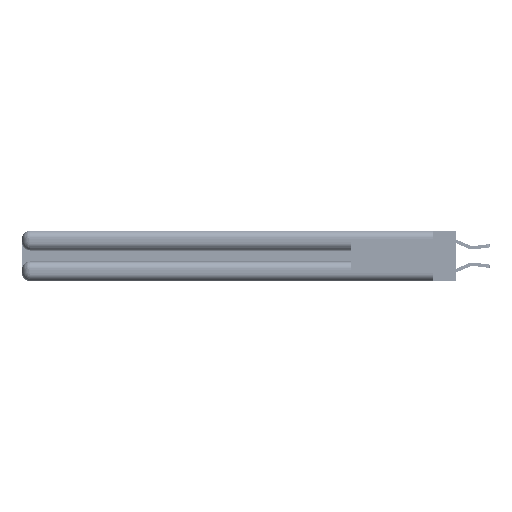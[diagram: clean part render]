
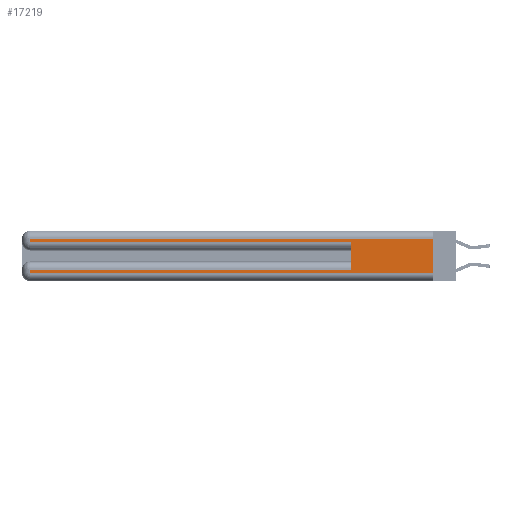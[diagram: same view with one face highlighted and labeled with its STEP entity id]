
A CAD part, left-side view. The second image highlights one B-rep face of the part: STEP entity #17219.
In plain terms, the highlighted planar face has unit normal (-1, 0, 0).
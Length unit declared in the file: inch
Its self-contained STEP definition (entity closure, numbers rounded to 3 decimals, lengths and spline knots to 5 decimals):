
#567 = CARTESIAN_POINT ( 'NONE',  ( 0., 2.94, 0.06 ) ) ;
#1386 = ORIENTED_EDGE ( 'NONE', *, *, #13064, .T. ) ;
#1607 = CARTESIAN_POINT ( 'NONE',  ( 0., 0.6, 0.145 ) ) ;
#2056 = VECTOR ( 'NONE', #31576, 39.37008 ) ;
#3484 = DIRECTION ( 'NONE',  ( 0., 1., 0. ) ) ;
#3649 = DIRECTION ( 'NONE',  ( 1., 0., 0. ) ) ;
#3768 = VERTEX_POINT ( 'NONE', #10625 ) ;
#4222 = LINE ( 'NONE', #1607, #11592 ) ;
#4477 = ORIENTED_EDGE ( 'NONE', *, *, #33767, .T. ) ;
#4599 = DIRECTION ( 'NONE',  ( 0., 0., -1. ) ) ;
#4734 = ORIENTED_EDGE ( 'NONE', *, *, #36542, .T. ) ;
#5939 = LINE ( 'NONE', #31522, #25085 ) ;
#6443 = LINE ( 'NONE', #23136, #7907 ) ;
#6954 = VERTEX_POINT ( 'NONE', #567 ) ;
#7397 = CARTESIAN_POINT ( 'NONE',  ( 0., 0.6, 0.285 ) ) ;
#7907 = VECTOR ( 'NONE', #3484, 39.37008 ) ;
#9080 = DIRECTION ( 'NONE',  ( 0., -1., 0. ) ) ;
#9557 = FACE_OUTER_BOUND ( 'NONE', #30323, .T. ) ;
#10322 = CARTESIAN_POINT ( 'NONE',  ( 0., 0., 0.31 ) ) ;
#10553 = VERTEX_POINT ( 'NONE', #7397 ) ;
#10625 = CARTESIAN_POINT ( 'NONE',  ( 0., 0.6, 0.085 ) ) ;
#11592 = VECTOR ( 'NONE', #26823, 39.37008 ) ;
#11743 = LINE ( 'NONE', #28624, #2056 ) ;
#11820 = PLANE ( 'NONE',  #14605 ) ;
#12938 = LINE ( 'NONE', #10322, #17382 ) ;
#12982 = EDGE_CURVE ( 'NONE', #3768, #16182, #6443, .T. ) ;
#13064 = EDGE_CURVE ( 'NONE', #24752, #29821, #12938, .T. ) ;
#13301 = LINE ( 'NONE', #30186, #20770 ) ;
#14605 = AXIS2_PLACEMENT_3D ( 'NONE', #34790, #3649, #20668 ) ;
#15495 = DIRECTION ( 'NONE',  ( 0., -1., 0. ) ) ;
#16145 = EDGE_CURVE ( 'NONE', #25427, #10553, #16730, .T. ) ;
#16182 = VERTEX_POINT ( 'NONE', #29796 ) ;
#16185 = ORIENTED_EDGE ( 'NONE', *, *, #12982, .T. ) ;
#16730 = LINE ( 'NONE', #25079, #29385 ) ;
#16937 = ORIENTED_EDGE ( 'NONE', *, *, #35867, .F. ) ;
#17219 = ADVANCED_FACE ( 'NONE', ( #9557 ), #11820, .F. ) ;
#17382 = VECTOR ( 'NONE', #21626, 39.37008 ) ;
#20173 = CARTESIAN_POINT ( 'NONE',  ( 0., 2.94, 0.31 ) ) ;
#20558 = CARTESIAN_POINT ( 'NONE',  ( 0., 2.94, 0.285 ) ) ;
#20668 = DIRECTION ( 'NONE',  ( 0., 0., -1. ) ) ;
#20770 = VECTOR ( 'NONE', #4599, 39.37008 ) ;
#21626 = DIRECTION ( 'NONE',  ( 0., 1., 0. ) ) ;
#21964 = CARTESIAN_POINT ( 'NONE',  ( 0., 0., 0.06 ) ) ;
#23136 = CARTESIAN_POINT ( 'NONE',  ( 0., 0., 0.085 ) ) ;
#24752 = VERTEX_POINT ( 'NONE', #34762 ) ;
#25079 = CARTESIAN_POINT ( 'NONE',  ( 0., 0., 0.285 ) ) ;
#25085 = VECTOR ( 'NONE', #9080, 39.37008 ) ;
#25427 = VERTEX_POINT ( 'NONE', #20558 ) ;
#25867 = CARTESIAN_POINT ( 'NONE',  ( 0., 2.94, 0.37 ) ) ;
#26823 = DIRECTION ( 'NONE',  ( 0., 0., 1. ) ) ;
#28177 = VECTOR ( 'NONE', #31078, 39.37008 ) ;
#28624 = CARTESIAN_POINT ( 'NONE',  ( 0., 2.94, 0.37 ) ) ;
#28685 = EDGE_CURVE ( 'NONE', #24752, #30561, #13301, .T. ) ;
#29385 = VECTOR ( 'NONE', #15495, 39.37008 ) ;
#29796 = CARTESIAN_POINT ( 'NONE',  ( 0., 2.94, 0.085 ) ) ;
#29821 = VERTEX_POINT ( 'NONE', #20173 ) ;
#30186 = CARTESIAN_POINT ( 'NONE',  ( 0., 0., 0.37 ) ) ;
#30323 = EDGE_LOOP ( 'NONE', ( #32486, #1386, #31373, #36296, #16937, #16185, #4734, #4477 ) ) ;
#30561 = VERTEX_POINT ( 'NONE', #21964 ) ;
#31078 = DIRECTION ( 'NONE',  ( 0., 0., -1. ) ) ;
#31373 = ORIENTED_EDGE ( 'NONE', *, *, #36070, .T. ) ;
#31522 = CARTESIAN_POINT ( 'NONE',  ( 0., 0., 0.06 ) ) ;
#31576 = DIRECTION ( 'NONE',  ( 0., 0., -1. ) ) ;
#32486 = ORIENTED_EDGE ( 'NONE', *, *, #28685, .F. ) ;
#33767 = EDGE_CURVE ( 'NONE', #6954, #30561, #5939, .T. ) ;
#34759 = LINE ( 'NONE', #25867, #28177 ) ;
#34762 = CARTESIAN_POINT ( 'NONE',  ( 0., 0., 0.31 ) ) ;
#34790 = CARTESIAN_POINT ( 'NONE',  ( 0., 0., 0.37 ) ) ;
#35867 = EDGE_CURVE ( 'NONE', #3768, #10553, #4222, .T. ) ;
#36070 = EDGE_CURVE ( 'NONE', #29821, #25427, #34759, .T. ) ;
#36296 = ORIENTED_EDGE ( 'NONE', *, *, #16145, .T. ) ;
#36542 = EDGE_CURVE ( 'NONE', #16182, #6954, #11743, .T. ) ;
